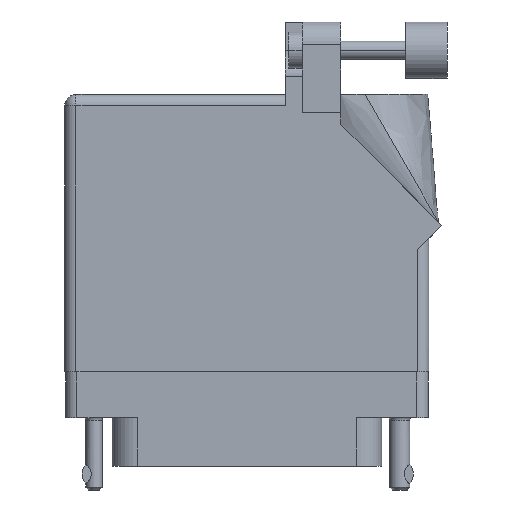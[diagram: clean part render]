
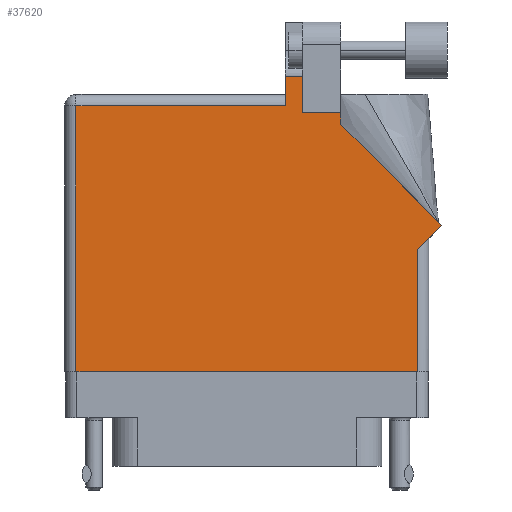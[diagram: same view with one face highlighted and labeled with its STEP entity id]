
A CAD part, front view. The second image highlights one B-rep face of the part: STEP entity #37620.
In plain terms, the highlighted face is planar.
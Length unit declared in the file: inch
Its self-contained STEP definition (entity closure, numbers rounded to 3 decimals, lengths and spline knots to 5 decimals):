
#55 = VERTEX_POINT ( 'NONE', #32675 ) ;
#319 = VECTOR ( 'NONE', #8317, 39.37008 ) ;
#3466 = LINE ( 'NONE', #17169, #22626 ) ;
#3741 = CARTESIAN_POINT ( 'NONE',  ( 0.212, 1.368, 0.455 ) ) ;
#4234 = ORIENTED_EDGE ( 'NONE', *, *, #26956, .T. ) ;
#4861 = CARTESIAN_POINT ( 'NONE',  ( 0.519, 1.26442, 0.455 ) ) ;
#4971 = VECTOR ( 'NONE', #16181, 39.37008 ) ;
#5079 = VERTEX_POINT ( 'NONE', #4861 ) ;
#6221 = LINE ( 'NONE', #20511, #319 ) ;
#6663 = DIRECTION ( 'NONE',  ( -1., 0., 0. ) ) ;
#6990 = EDGE_CURVE ( 'NONE', #43860, #11260, #36824, .T. ) ;
#7689 = EDGE_CURVE ( 'NONE', #5079, #48907, #30744, .T. ) ;
#7758 = CARTESIAN_POINT ( 'NONE',  ( 0.212, 1.43, 0.455 ) ) ;
#8034 = EDGE_CURVE ( 'NONE', #48907, #36581, #43348, .T. ) ;
#8317 = DIRECTION ( 'NONE',  ( 0., 1., 0. ) ) ;
#8556 = VERTEX_POINT ( 'NONE', #11335 ) ;
#9111 = LINE ( 'NONE', #48973, #20461 ) ;
#9733 = EDGE_CURVE ( 'NONE', #24631, #8556, #26316, .T. ) ;
#10602 = EDGE_CURVE ( 'NONE', #8556, #38388, #3466, .T. ) ;
#11260 = VERTEX_POINT ( 'NONE', #3741 ) ;
#11335 = CARTESIAN_POINT ( 'NONE',  ( -0.943, -0.1, 0.455 ) ) ;
#11344 = FACE_OUTER_BOUND ( 'NONE', #32031, .T. ) ;
#11487 = PLANE ( 'NONE',  #21664 ) ;
#12723 = CARTESIAN_POINT ( 'NONE',  ( 0.519, 1.33, 0.455 ) ) ;
#12880 = CARTESIAN_POINT ( 'NONE',  ( 1.005, 0.637, 0.455 ) ) ;
#13536 = EDGE_CURVE ( 'NONE', #11260, #24631, #20593, .T. ) ;
#13835 = CARTESIAN_POINT ( 'NONE',  ( 0.519, 1.33, 0.455 ) ) ;
#14000 = VECTOR ( 'NONE', #46501, 39.37008 ) ;
#14954 = DIRECTION ( 'NONE',  ( 0., -1., 0. ) ) ;
#15667 = DIRECTION ( 'NONE',  ( 0., 0., -1. ) ) ;
#16064 = CARTESIAN_POINT ( 'NONE',  ( 0.943, 0.575, 0.455 ) ) ;
#16181 = DIRECTION ( 'NONE',  ( 0., 1., 0. ) ) ;
#16486 = VERTEX_POINT ( 'NONE', #45655 ) ;
#16952 = ORIENTED_EDGE ( 'NONE', *, *, #8034, .T. ) ;
#17169 = CARTESIAN_POINT ( 'NONE',  ( -1.005, -0.1, 0.455 ) ) ;
#17443 = EDGE_CURVE ( 'NONE', #55, #5079, #34695, .T. ) ;
#18151 = LINE ( 'NONE', #12880, #31371 ) ;
#20162 = EDGE_CURVE ( 'NONE', #47808, #55, #18151, .T. ) ;
#20461 = VECTOR ( 'NONE', #48623, 39.37008 ) ;
#20511 = CARTESIAN_POINT ( 'NONE',  ( 0.306, 1.33, 0.455 ) ) ;
#20593 = LINE ( 'NONE', #25792, #41643 ) ;
#20831 = CARTESIAN_POINT ( 'NONE',  ( 0.306, 1.33, 0.455 ) ) ;
#21664 = AXIS2_PLACEMENT_3D ( 'NONE', #34969, #15667, #23380 ) ;
#21972 = CARTESIAN_POINT ( 'NONE',  ( -0.943, -0.1, 0.455 ) ) ;
#22626 = VECTOR ( 'NONE', #40538, 39.37008 ) ;
#22938 = CARTESIAN_POINT ( 'NONE',  ( 1.07571, 0.70771, 0.455 ) ) ;
#23380 = DIRECTION ( 'NONE',  ( -1., 0., 0. ) ) ;
#23920 = VECTOR ( 'NONE', #14954, 39.37008 ) ;
#24631 = VERTEX_POINT ( 'NONE', #29385 ) ;
#25721 = DIRECTION ( 'NONE',  ( -1., 0., 0. ) ) ;
#25792 = CARTESIAN_POINT ( 'NONE',  ( -1.005, 1.368, 0.455 ) ) ;
#26316 = LINE ( 'NONE', #21972, #23920 ) ;
#26956 = EDGE_CURVE ( 'NONE', #36581, #16486, #6221, .T. ) ;
#28640 = ORIENTED_EDGE ( 'NONE', *, *, #6990, .T. ) ;
#29385 = CARTESIAN_POINT ( 'NONE',  ( -0.943, 1.368, 0.455 ) ) ;
#29998 = CARTESIAN_POINT ( 'NONE',  ( 0.943, -0.1, 0.455 ) ) ;
#30544 = ORIENTED_EDGE ( 'NONE', *, *, #20162, .T. ) ;
#30744 = LINE ( 'NONE', #35170, #4971 ) ;
#30832 = DIRECTION ( 'NONE',  ( -0.707, 0.707, 0. ) ) ;
#31220 = ORIENTED_EDGE ( 'NONE', *, *, #41706, .T. ) ;
#31371 = VECTOR ( 'NONE', #40914, 39.37008 ) ;
#31678 = ORIENTED_EDGE ( 'NONE', *, *, #10602, .T. ) ;
#32031 = EDGE_LOOP ( 'NONE', ( #4234, #31220, #28640, #42451, #36482, #31678, #42229, #30544, #44491, #48962, #16952 ) ) ;
#32675 = CARTESIAN_POINT ( 'NONE',  ( 1.07571, 0.70771, 0.455 ) ) ;
#32845 = VECTOR ( 'NONE', #30832, 39.37008 ) ;
#34695 = LINE ( 'NONE', #22938, #32845 ) ;
#34969 = CARTESIAN_POINT ( 'NONE',  ( -1.005, 1.43, 0.455 ) ) ;
#35170 = CARTESIAN_POINT ( 'NONE',  ( 0.519, 1.26442, 0.455 ) ) ;
#35529 = VECTOR ( 'NONE', #25721, 39.37008 ) ;
#35850 = EDGE_CURVE ( 'NONE', #38388, #47808, #9111, .T. ) ;
#36482 = ORIENTED_EDGE ( 'NONE', *, *, #9733, .T. ) ;
#36581 = VERTEX_POINT ( 'NONE', #20831 ) ;
#36824 = LINE ( 'NONE', #7758, #14000 ) ;
#37620 = ADVANCED_FACE ( 'NONE', ( #11344 ), #11487, .F. ) ;
#38388 = VERTEX_POINT ( 'NONE', #29998 ) ;
#40538 = DIRECTION ( 'NONE',  ( 1., 0., 0. ) ) ;
#40914 = DIRECTION ( 'NONE',  ( 0.707, 0.707, 0. ) ) ;
#41105 = LINE ( 'NONE', #44808, #44677 ) ;
#41643 = VECTOR ( 'NONE', #6663, 39.37008 ) ;
#41706 = EDGE_CURVE ( 'NONE', #16486, #43860, #41105, .T. ) ;
#42229 = ORIENTED_EDGE ( 'NONE', *, *, #35850, .T. ) ;
#42451 = ORIENTED_EDGE ( 'NONE', *, *, #13536, .T. ) ;
#43348 = LINE ( 'NONE', #13835, #35529 ) ;
#43860 = VERTEX_POINT ( 'NONE', #44130 ) ;
#44130 = CARTESIAN_POINT ( 'NONE',  ( 0.212, 1.5315, 0.455 ) ) ;
#44491 = ORIENTED_EDGE ( 'NONE', *, *, #17443, .T. ) ;
#44677 = VECTOR ( 'NONE', #49005, 39.37008 ) ;
#44808 = CARTESIAN_POINT ( 'NONE',  ( 0.63677, 1.5315, 0.455 ) ) ;
#45655 = CARTESIAN_POINT ( 'NONE',  ( 0.306, 1.5315, 0.455 ) ) ;
#46501 = DIRECTION ( 'NONE',  ( 0., -1., 0. ) ) ;
#47808 = VERTEX_POINT ( 'NONE', #16064 ) ;
#48623 = DIRECTION ( 'NONE',  ( 0., 1., 0. ) ) ;
#48907 = VERTEX_POINT ( 'NONE', #12723 ) ;
#48962 = ORIENTED_EDGE ( 'NONE', *, *, #7689, .T. ) ;
#48973 = CARTESIAN_POINT ( 'NONE',  ( 0.943, 0.637, 0.455 ) ) ;
#49005 = DIRECTION ( 'NONE',  ( -1., 0., 0. ) ) ;
